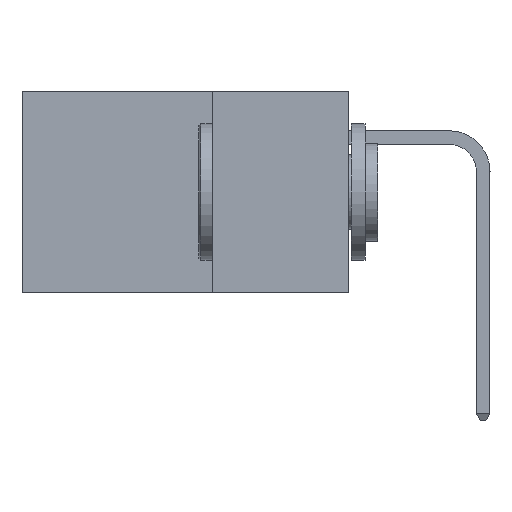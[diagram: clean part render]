
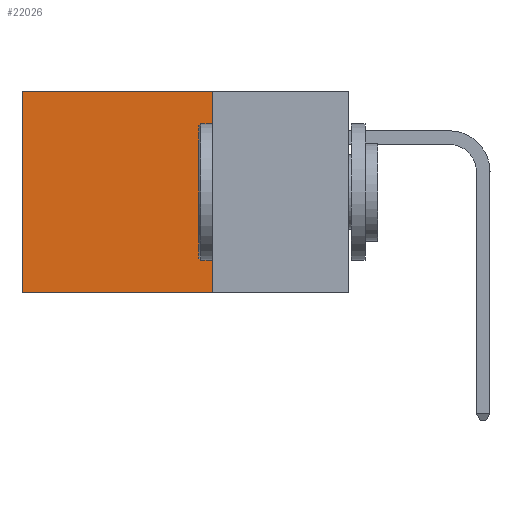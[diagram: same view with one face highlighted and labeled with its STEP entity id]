
A CAD part, left-side view. The second image highlights one B-rep face of the part: STEP entity #22026.
In plain terms, the highlighted planar face has unit normal (-1, 0, 0).
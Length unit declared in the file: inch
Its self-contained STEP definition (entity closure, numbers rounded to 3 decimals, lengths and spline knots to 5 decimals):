
#171 = FACE_OUTER_BOUND ( 'NONE', #30901, .T. ) ;
#2383 = LINE ( 'NONE', #20903, #11998 ) ;
#4725 = AXIS2_PLACEMENT_3D ( 'NONE', #12206, #37293, #15800 ) ;
#5232 = EDGE_CURVE ( 'NONE', #46319, #15516, #2383, .T. ) ;
#5961 = DIRECTION ( 'NONE',  ( 0., 0., -1. ) ) ;
#8472 = VECTOR ( 'NONE', #24810, 39.37008 ) ;
#10531 = CARTESIAN_POINT ( 'NONE',  ( 0.2875, 0.25, 0. ) ) ;
#11568 = ORIENTED_EDGE ( 'NONE', *, *, #30056, .T. ) ;
#11998 = VECTOR ( 'NONE', #13693, 39.37008 ) ;
#12206 = CARTESIAN_POINT ( 'NONE',  ( 0.2875, 0.25, 0. ) ) ;
#13693 = DIRECTION ( 'NONE',  ( 0., 1., 0. ) ) ;
#14775 = EDGE_CURVE ( 'NONE', #38029, #39110, #27560, .T. ) ;
#15516 = VERTEX_POINT ( 'NONE', #26002 ) ;
#15800 = DIRECTION ( 'NONE',  ( 0., 0., -1. ) ) ;
#17554 = CARTESIAN_POINT ( 'NONE',  ( 0.2875, 0.25, 0. ) ) ;
#19508 = VECTOR ( 'NONE', #5961, 39.37008 ) ;
#19762 = CARTESIAN_POINT ( 'NONE',  ( 0.2875, 0.25, 0. ) ) ;
#19893 = EDGE_CURVE ( 'NONE', #38029, #46319, #28419, .T. ) ;
#20903 = CARTESIAN_POINT ( 'NONE',  ( 0.2875, 0.25, -0.37 ) ) ;
#21114 = ORIENTED_EDGE ( 'NONE', *, *, #19893, .F. ) ;
#22026 = ADVANCED_FACE ( 'NONE', ( #171 ), #26450, .F. ) ;
#22626 = CARTESIAN_POINT ( 'NONE',  ( 0.2875, 0.25, -0.37 ) ) ;
#24810 = DIRECTION ( 'NONE',  ( 0., 1., 0. ) ) ;
#24890 = ORIENTED_EDGE ( 'NONE', *, *, #14775, .T. ) ;
#25286 = CARTESIAN_POINT ( 'NONE',  ( 0.2875, 0.6, 0. ) ) ;
#26002 = CARTESIAN_POINT ( 'NONE',  ( 0.2875, 0.6, -0.37 ) ) ;
#26450 = PLANE ( 'NONE',  #4725 ) ;
#27025 = ORIENTED_EDGE ( 'NONE', *, *, #5232, .F. ) ;
#27302 = VECTOR ( 'NONE', #41231, 39.37008 ) ;
#27560 = LINE ( 'NONE', #10531, #8472 ) ;
#28419 = LINE ( 'NONE', #19762, #27302 ) ;
#30056 = EDGE_CURVE ( 'NONE', #39110, #15516, #39702, .T. ) ;
#30901 = EDGE_LOOP ( 'NONE', ( #11568, #27025, #21114, #24890 ) ) ;
#37293 = DIRECTION ( 'NONE',  ( 1., 0., 0. ) ) ;
#38029 = VERTEX_POINT ( 'NONE', #17554 ) ;
#38296 = CARTESIAN_POINT ( 'NONE',  ( 0.2875, 0.6, 0. ) ) ;
#39110 = VERTEX_POINT ( 'NONE', #25286 ) ;
#39702 = LINE ( 'NONE', #38296, #19508 ) ;
#41231 = DIRECTION ( 'NONE',  ( 0., 0., -1. ) ) ;
#46319 = VERTEX_POINT ( 'NONE', #22626 ) ;
